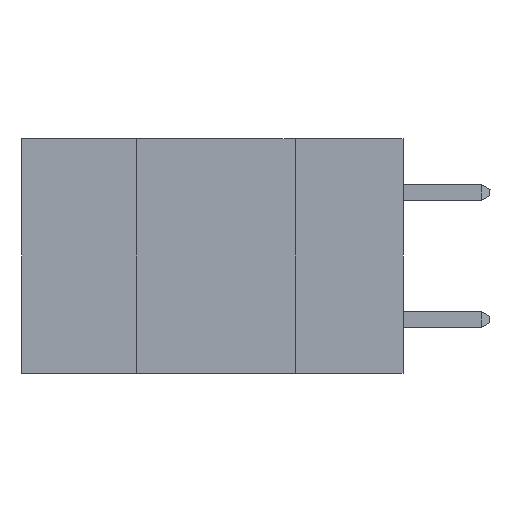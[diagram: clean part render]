
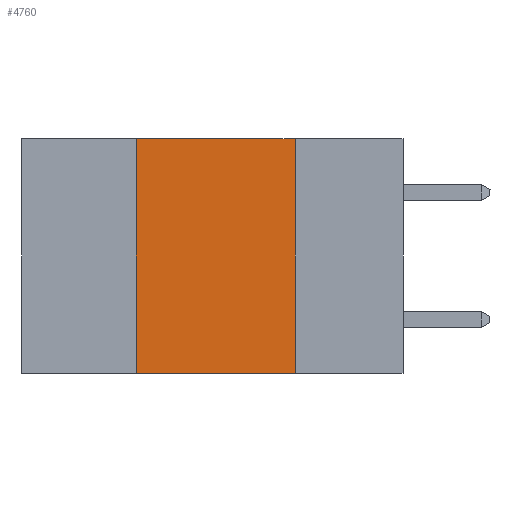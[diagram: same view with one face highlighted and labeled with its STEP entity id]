
A CAD part, left-side view. The second image highlights one B-rep face of the part: STEP entity #4760.
In plain terms, the highlighted planar face has unit normal (-1, 0, 0).
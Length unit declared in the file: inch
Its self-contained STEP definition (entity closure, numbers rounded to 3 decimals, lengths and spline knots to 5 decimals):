
#230 = DIRECTION ( 'NONE',  ( 1., 0., 0. ) ) ;
#708 = EDGE_CURVE ( 'NONE', #14898, #16239, #14808, .T. ) ;
#920 = EDGE_CURVE ( 'NONE', #21401, #14898, #1738, .T. ) ;
#1254 = VERTEX_POINT ( 'NONE', #4704 ) ;
#1738 = LINE ( 'NONE', #14238, #13292 ) ;
#2238 = EDGE_CURVE ( 'NONE', #16239, #1254, #16537, .T. ) ;
#3599 = ORIENTED_EDGE ( 'NONE', *, *, #708, .F. ) ;
#4042 = DIRECTION ( 'NONE',  ( 0., -1., 0. ) ) ;
#4242 = DIRECTION ( 'NONE',  ( 0., 0., -1. ) ) ;
#4279 = VECTOR ( 'NONE', #9380, 39.37008 ) ;
#4704 = CARTESIAN_POINT ( 'NONE',  ( 0., 0.17, -0.37 ) ) ;
#4751 = AXIS2_PLACEMENT_3D ( 'NONE', #19811, #230, #4242 ) ;
#4760 = ADVANCED_FACE ( 'NONE', ( #24398 ), #15770, .F. ) ;
#4782 = VECTOR ( 'NONE', #4042, 39.37008 ) ;
#6574 = EDGE_CURVE ( 'NONE', #21401, #1254, #23777, .T. ) ;
#7646 = CARTESIAN_POINT ( 'NONE',  ( 0., 0.42, 0. ) ) ;
#8170 = CARTESIAN_POINT ( 'NONE',  ( 0., 0.17, 0. ) ) ;
#9380 = DIRECTION ( 'NONE',  ( 0., -1., 0. ) ) ;
#13292 = VECTOR ( 'NONE', #24077, 39.37008 ) ;
#14238 = CARTESIAN_POINT ( 'NONE',  ( 0., 0.42, 0. ) ) ;
#14642 = ORIENTED_EDGE ( 'NONE', *, *, #6574, .T. ) ;
#14808 = LINE ( 'NONE', #23142, #4782 ) ;
#14898 = VERTEX_POINT ( 'NONE', #7646 ) ;
#15770 = PLANE ( 'NONE',  #4751 ) ;
#16193 = VECTOR ( 'NONE', #22785, 39.37008 ) ;
#16239 = VERTEX_POINT ( 'NONE', #8170 ) ;
#16537 = LINE ( 'NONE', #16886, #16193 ) ;
#16886 = CARTESIAN_POINT ( 'NONE',  ( 0., 0.17, 0. ) ) ;
#19811 = CARTESIAN_POINT ( 'NONE',  ( 0., 0.6, 0. ) ) ;
#21382 = CARTESIAN_POINT ( 'NONE',  ( 0., 0.6, -0.37 ) ) ;
#21401 = VERTEX_POINT ( 'NONE', #22397 ) ;
#21954 = EDGE_LOOP ( 'NONE', ( #24140, #3599, #22551, #14642 ) ) ;
#22397 = CARTESIAN_POINT ( 'NONE',  ( 0., 0.42, -0.37 ) ) ;
#22551 = ORIENTED_EDGE ( 'NONE', *, *, #920, .F. ) ;
#22785 = DIRECTION ( 'NONE',  ( 0., 0., -1. ) ) ;
#23142 = CARTESIAN_POINT ( 'NONE',  ( 0., 0.6, 0. ) ) ;
#23777 = LINE ( 'NONE', #21382, #4279 ) ;
#24077 = DIRECTION ( 'NONE',  ( 0., 0., 1. ) ) ;
#24140 = ORIENTED_EDGE ( 'NONE', *, *, #2238, .F. ) ;
#24398 = FACE_OUTER_BOUND ( 'NONE', #21954, .T. ) ;
